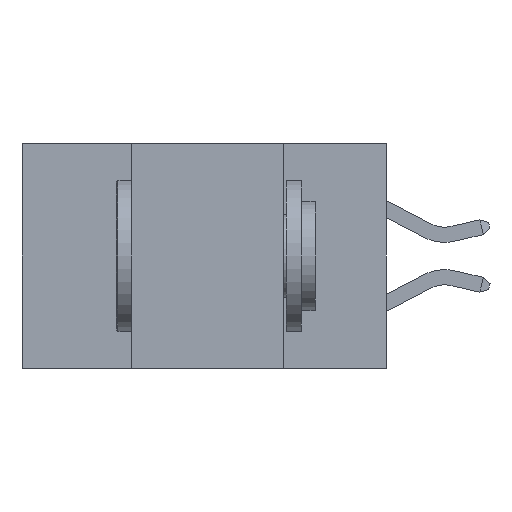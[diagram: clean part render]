
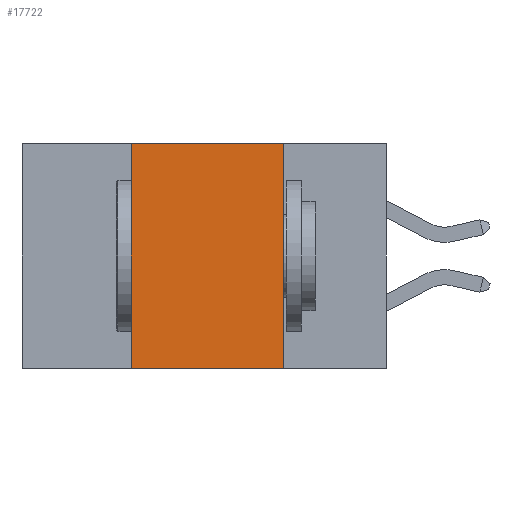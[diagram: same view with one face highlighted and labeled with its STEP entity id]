
A CAD part, left-side view. The second image highlights one B-rep face of the part: STEP entity #17722.
In plain terms, the highlighted planar face has unit normal (-1, 0, 0).
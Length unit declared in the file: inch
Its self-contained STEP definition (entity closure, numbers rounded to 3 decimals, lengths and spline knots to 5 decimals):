
#1335 = CARTESIAN_POINT ( 'NONE',  ( 0., 0.6, 0. ) ) ;
#2750 = VERTEX_POINT ( 'NONE', #12959 ) ;
#3473 = CARTESIAN_POINT ( 'NONE',  ( 0., 0.17, -0.37 ) ) ;
#4233 = LINE ( 'NONE', #10852, #8495 ) ;
#4776 = VERTEX_POINT ( 'NONE', #3473 ) ;
#5714 = DIRECTION ( 'NONE',  ( 0., -1., 0. ) ) ;
#6021 = PLANE ( 'NONE',  #11565 ) ;
#6361 = LINE ( 'NONE', #15156, #20237 ) ;
#6787 = ORIENTED_EDGE ( 'NONE', *, *, #20182, .T. ) ;
#7317 = EDGE_CURVE ( 'NONE', #16402, #8618, #7464, .T. ) ;
#7464 = LINE ( 'NONE', #13282, #19384 ) ;
#7627 = CARTESIAN_POINT ( 'NONE',  ( 0., 0.6, 0. ) ) ;
#7798 = ORIENTED_EDGE ( 'NONE', *, *, #9407, .F. ) ;
#8337 = VECTOR ( 'NONE', #12458, 39.37008 ) ;
#8495 = VECTOR ( 'NONE', #18624, 39.37008 ) ;
#8534 = DIRECTION ( 'NONE',  ( 0., 0., 1. ) ) ;
#8618 = VERTEX_POINT ( 'NONE', #18340 ) ;
#9407 = EDGE_CURVE ( 'NONE', #8618, #2750, #12002, .T. ) ;
#10751 = DIRECTION ( 'NONE',  ( 0., 0., -1. ) ) ;
#10852 = CARTESIAN_POINT ( 'NONE',  ( 0., 0.17, -0.37 ) ) ;
#11565 = AXIS2_PLACEMENT_3D ( 'NONE', #7627, #20032, #10751 ) ;
#12002 = LINE ( 'NONE', #1335, #8337 ) ;
#12169 = EDGE_CURVE ( 'NONE', #2750, #4776, #4233, .T. ) ;
#12458 = DIRECTION ( 'NONE',  ( 0., -1., 0. ) ) ;
#12947 = CARTESIAN_POINT ( 'NONE',  ( 0., 0.42, -0.37 ) ) ;
#12959 = CARTESIAN_POINT ( 'NONE',  ( 0., 0.17, 0. ) ) ;
#13282 = CARTESIAN_POINT ( 'NONE',  ( 0., 0.42, -0.37 ) ) ;
#15156 = CARTESIAN_POINT ( 'NONE',  ( 0., 0.6, -0.37 ) ) ;
#15171 = ORIENTED_EDGE ( 'NONE', *, *, #7317, .F. ) ;
#15787 = EDGE_LOOP ( 'NONE', ( #20170, #7798, #15171, #6787 ) ) ;
#16402 = VERTEX_POINT ( 'NONE', #12947 ) ;
#17722 = ADVANCED_FACE ( 'NONE', ( #20108 ), #6021, .F. ) ;
#18340 = CARTESIAN_POINT ( 'NONE',  ( 0., 0.42, 0. ) ) ;
#18624 = DIRECTION ( 'NONE',  ( 0., 0., -1. ) ) ;
#19384 = VECTOR ( 'NONE', #8534, 39.37008 ) ;
#20032 = DIRECTION ( 'NONE',  ( 1., 0., 0. ) ) ;
#20108 = FACE_OUTER_BOUND ( 'NONE', #15787, .T. ) ;
#20170 = ORIENTED_EDGE ( 'NONE', *, *, #12169, .F. ) ;
#20182 = EDGE_CURVE ( 'NONE', #16402, #4776, #6361, .T. ) ;
#20237 = VECTOR ( 'NONE', #5714, 39.37008 ) ;
